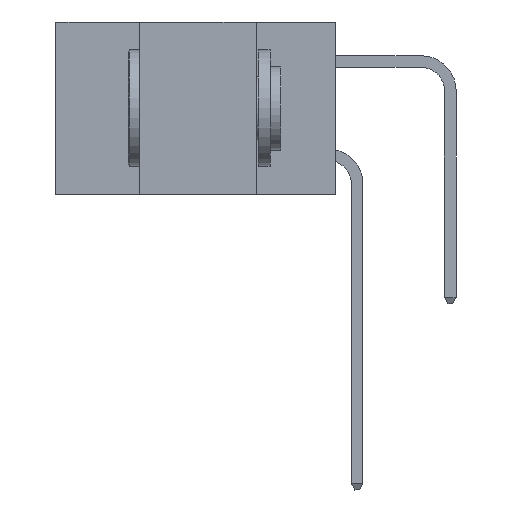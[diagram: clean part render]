
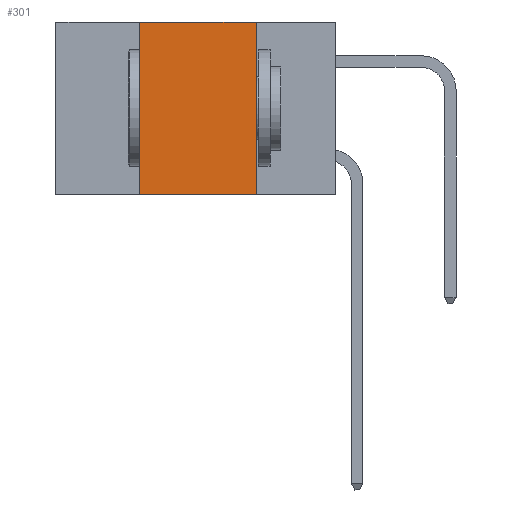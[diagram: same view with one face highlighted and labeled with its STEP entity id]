
A CAD part, left-side view. The second image highlights one B-rep face of the part: STEP entity #301.
In plain terms, the highlighted planar face has unit normal (-1, 0, 0).
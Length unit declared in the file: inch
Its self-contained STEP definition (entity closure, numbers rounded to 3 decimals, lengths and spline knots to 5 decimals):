
#301 = ADVANCED_FACE ( 'NONE', ( #5673 ), #9676, .F. ) ;
#869 = VERTEX_POINT ( 'NONE', #13064 ) ;
#1223 = ORIENTED_EDGE ( 'NONE', *, *, #8474, .T. ) ;
#1630 = CARTESIAN_POINT ( 'NONE',  ( 0., 0.42, -0.37 ) ) ;
#1752 = DIRECTION ( 'NONE',  ( 0., 0., -1. ) ) ;
#2397 = CARTESIAN_POINT ( 'NONE',  ( 0., 0.17, 0. ) ) ;
#2809 = CARTESIAN_POINT ( 'NONE',  ( 0., 0.6, 0. ) ) ;
#2903 = CARTESIAN_POINT ( 'NONE',  ( 0., 0.17, 0. ) ) ;
#3105 = ORIENTED_EDGE ( 'NONE', *, *, #6749, .F. ) ;
#3422 = LINE ( 'NONE', #2809, #19493 ) ;
#4600 = DIRECTION ( 'NONE',  ( 0., 0., -1. ) ) ;
#4764 = LINE ( 'NONE', #6140, #15192 ) ;
#5047 = DIRECTION ( 'NONE',  ( 1., 0., 0. ) ) ;
#5673 = FACE_OUTER_BOUND ( 'NONE', #9770, .T. ) ;
#6140 = CARTESIAN_POINT ( 'NONE',  ( 0., 0.42, 0. ) ) ;
#6749 = EDGE_CURVE ( 'NONE', #17589, #9081, #4764, .T. ) ;
#7247 = AXIS2_PLACEMENT_3D ( 'NONE', #19287, #5047, #1752 ) ;
#7416 = CARTESIAN_POINT ( 'NONE',  ( 0., 0.6, -0.37 ) ) ;
#8405 = VECTOR ( 'NONE', #15430, 39.37008 ) ;
#8474 = EDGE_CURVE ( 'NONE', #17589, #869, #11370, .T. ) ;
#9081 = VERTEX_POINT ( 'NONE', #17440 ) ;
#9503 = ORIENTED_EDGE ( 'NONE', *, *, #10658, .F. ) ;
#9676 = PLANE ( 'NONE',  #7247 ) ;
#9770 = EDGE_LOOP ( 'NONE', ( #9503, #10597, #3105, #1223 ) ) ;
#10597 = ORIENTED_EDGE ( 'NONE', *, *, #14168, .F. ) ;
#10658 = EDGE_CURVE ( 'NONE', #12803, #869, #13522, .T. ) ;
#11370 = LINE ( 'NONE', #7416, #8405 ) ;
#12803 = VERTEX_POINT ( 'NONE', #2397 ) ;
#13064 = CARTESIAN_POINT ( 'NONE',  ( 0., 0.17, -0.37 ) ) ;
#13522 = LINE ( 'NONE', #2903, #18505 ) ;
#14168 = EDGE_CURVE ( 'NONE', #9081, #12803, #3422, .T. ) ;
#14762 = DIRECTION ( 'NONE',  ( 0., 0., 1. ) ) ;
#15192 = VECTOR ( 'NONE', #14762, 39.37008 ) ;
#15430 = DIRECTION ( 'NONE',  ( 0., -1., 0. ) ) ;
#16972 = DIRECTION ( 'NONE',  ( 0., -1., 0. ) ) ;
#17440 = CARTESIAN_POINT ( 'NONE',  ( 0., 0.42, 0. ) ) ;
#17589 = VERTEX_POINT ( 'NONE', #1630 ) ;
#18505 = VECTOR ( 'NONE', #4600, 39.37008 ) ;
#19287 = CARTESIAN_POINT ( 'NONE',  ( 0., 0.6, 0. ) ) ;
#19493 = VECTOR ( 'NONE', #16972, 39.37008 ) ;
